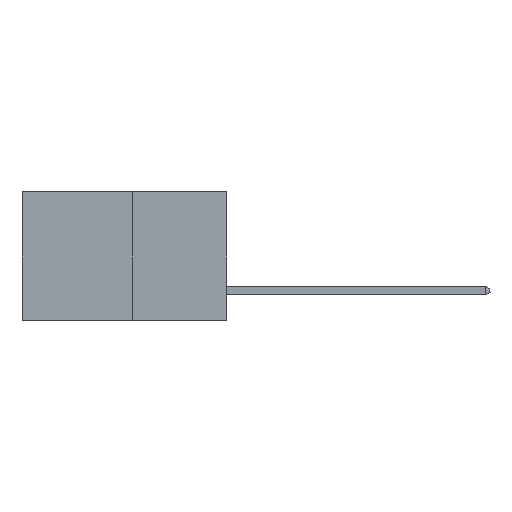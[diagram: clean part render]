
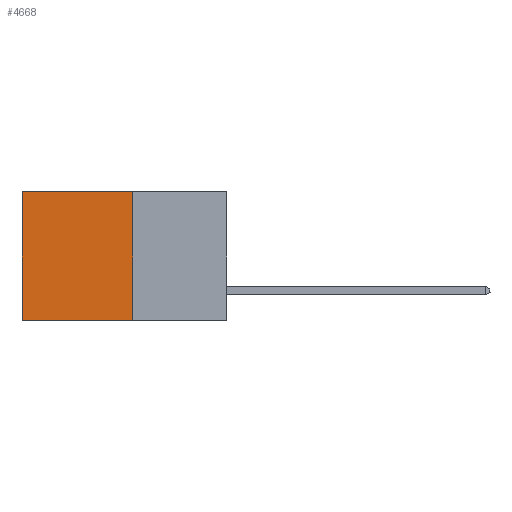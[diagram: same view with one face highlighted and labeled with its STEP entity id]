
A CAD part, left-side view. The second image highlights one B-rep face of the part: STEP entity #4668.
In plain terms, the highlighted planar face has unit normal (-1, 0, 0).
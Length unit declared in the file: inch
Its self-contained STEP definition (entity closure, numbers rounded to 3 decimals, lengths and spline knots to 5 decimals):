
#1970 = EDGE_CURVE ( 'NONE', #4659, #16585, #23329, .T. ) ;
#2076 = LINE ( 'NONE', #8582, #19427 ) ;
#2720 = VECTOR ( 'NONE', #26711, 39.37008 ) ;
#3438 = CARTESIAN_POINT ( 'NONE',  ( 0.277, 0.27, -0.37 ) ) ;
#3508 = CARTESIAN_POINT ( 'NONE',  ( 0.277, 0.27, -0.37 ) ) ;
#4659 = VERTEX_POINT ( 'NONE', #20297 ) ;
#4668 = ADVANCED_FACE ( 'NONE', ( #32304 ), #24116, .F. ) ;
#5315 = LINE ( 'NONE', #3508, #18230 ) ;
#5989 = DIRECTION ( 'NONE',  ( 0., 0., -1. ) ) ;
#8582 = CARTESIAN_POINT ( 'NONE',  ( 0.277, 0.59, -0.37 ) ) ;
#9551 = ORIENTED_EDGE ( 'NONE', *, *, #14981, .T. ) ;
#11157 = LINE ( 'NONE', #29168, #25738 ) ;
#11254 = CARTESIAN_POINT ( 'NONE',  ( 0.277, 0.27, -0.37 ) ) ;
#13217 = VERTEX_POINT ( 'NONE', #30541 ) ;
#13762 = DIRECTION ( 'NONE',  ( 0., 1., 0. ) ) ;
#14981 = EDGE_CURVE ( 'NONE', #4659, #13217, #11157, .T. ) ;
#16046 = AXIS2_PLACEMENT_3D ( 'NONE', #24001, #19278, #19274 ) ;
#16585 = VERTEX_POINT ( 'NONE', #3438 ) ;
#17611 = EDGE_LOOP ( 'NONE', ( #23429, #19920, #20462, #9551 ) ) ;
#18143 = VERTEX_POINT ( 'NONE', #32345 ) ;
#18230 = VECTOR ( 'NONE', #24171, 39.37008 ) ;
#19274 = DIRECTION ( 'NONE',  ( 0., 0., -1. ) ) ;
#19278 = DIRECTION ( 'NONE',  ( 1., 0., 0. ) ) ;
#19427 = VECTOR ( 'NONE', #5989, 39.37008 ) ;
#19920 = ORIENTED_EDGE ( 'NONE', *, *, #26908, .F. ) ;
#20297 = CARTESIAN_POINT ( 'NONE',  ( 0.277, 0.27, 0. ) ) ;
#20462 = ORIENTED_EDGE ( 'NONE', *, *, #1970, .F. ) ;
#21939 = EDGE_CURVE ( 'NONE', #13217, #18143, #2076, .T. ) ;
#23329 = LINE ( 'NONE', #11254, #2720 ) ;
#23429 = ORIENTED_EDGE ( 'NONE', *, *, #21939, .T. ) ;
#24001 = CARTESIAN_POINT ( 'NONE',  ( 0.277, 0.27, -0.37 ) ) ;
#24116 = PLANE ( 'NONE',  #16046 ) ;
#24171 = DIRECTION ( 'NONE',  ( 0., 1., 0. ) ) ;
#25738 = VECTOR ( 'NONE', #13762, 39.37008 ) ;
#26711 = DIRECTION ( 'NONE',  ( 0., 0., -1. ) ) ;
#26908 = EDGE_CURVE ( 'NONE', #16585, #18143, #5315, .T. ) ;
#29168 = CARTESIAN_POINT ( 'NONE',  ( 0.277, 0.27, 0. ) ) ;
#30541 = CARTESIAN_POINT ( 'NONE',  ( 0.277, 0.59, 0. ) ) ;
#32304 = FACE_OUTER_BOUND ( 'NONE', #17611, .T. ) ;
#32345 = CARTESIAN_POINT ( 'NONE',  ( 0.277, 0.59, -0.37 ) ) ;
